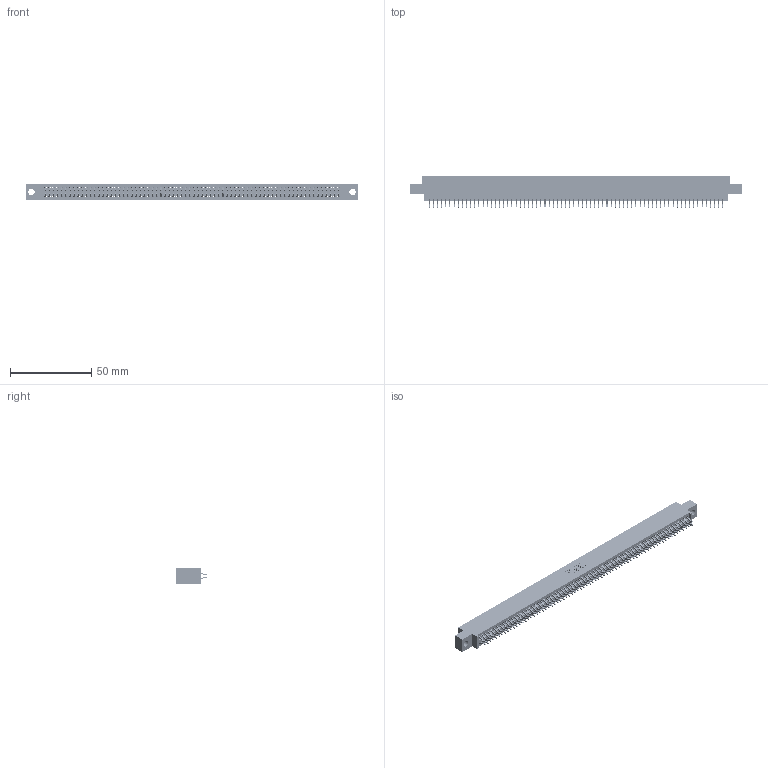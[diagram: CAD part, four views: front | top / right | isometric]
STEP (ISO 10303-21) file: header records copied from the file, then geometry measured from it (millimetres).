
FILE_DESCRIPTION (( 'STEP AP203' ), '1' );
FILE_NAME ('345-144-556-804.STEP', '2021-05-26T03:16:10', ( '' ), ( '' ), 'SwSTEP 2.0', 'SolidWorks 2020', '' );
FILE_SCHEMA (( 'CONFIG_CONTROL_DESIGN' ));
Length unit declared in the file: inch
Products named in the file (3): 345 Part_0.170 Offset - 0.156 Dia-TI; 345-144-556-804; 345-292-001_556 Tail
Assembly tree (145 placements, depth 2):
  345-144-556-804
    345 Part_0.170 Offset - 0.156 Dia-TI
    345-292-001_556 Tail  x144
Bounding box: 204.09 x 19.24 x 9.4 mm (x, y, z)
Volume: 19878.9 mm3; surface area: 29834.3 mm2
Topology: 145 solids, 145 shells, 8208 faces, 24437 edges, 16098 vertices
Faces by surface type: plane 5426, cylinder 2782
Entity records: 53225 total; most frequent: CARTESIAN_POINT 8914, ORIENTED_EDGE 8834, DIRECTION 7809, EDGE_CURVE 4417, LINE 3989, VECTOR 3989, VERTEX_POINT 2942, AXIS2_PLACEMENT_3D 1910
